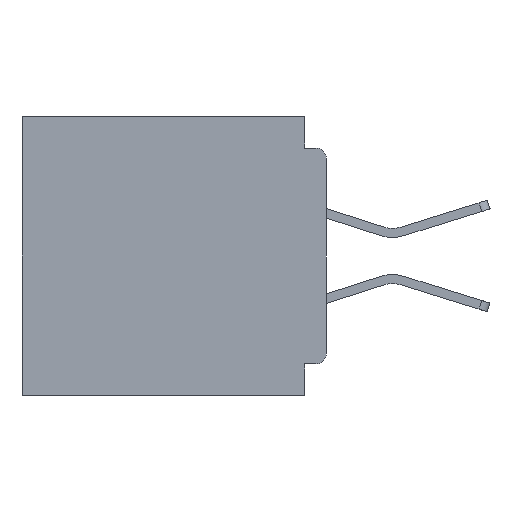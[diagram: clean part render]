
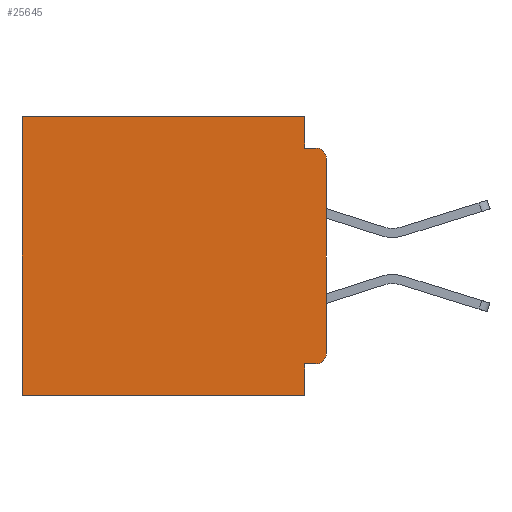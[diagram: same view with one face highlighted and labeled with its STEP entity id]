
A CAD part, left-side view. The second image highlights one B-rep face of the part: STEP entity #25645.
In plain terms, the highlighted planar face has unit normal (-1, 0, 0).
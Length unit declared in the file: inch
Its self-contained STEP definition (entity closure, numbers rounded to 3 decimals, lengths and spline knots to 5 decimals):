
#395 = FACE_OUTER_BOUND ( 'NONE', #23932, .T. ) ;
#599 = LINE ( 'NONE', #35341, #52289 ) ;
#626 = AXIS2_PLACEMENT_3D ( 'NONE', #2912, #31562, #7091 ) ;
#1434 = EDGE_CURVE ( 'NONE', #46200, #26288, #18118, .T. ) ;
#2071 = EDGE_CURVE ( 'NONE', #22953, #18484, #30755, .T. ) ;
#2912 = CARTESIAN_POINT ( 'NONE',  ( 0.3, 0.015, -0.34 ) ) ;
#4743 = ORIENTED_EDGE ( 'NONE', *, *, #30629, .F. ) ;
#5328 = VECTOR ( 'NONE', #30180, 39.37008 ) ;
#5553 = ORIENTED_EDGE ( 'NONE', *, *, #47998, .F. ) ;
#5701 = CARTESIAN_POINT ( 'NONE',  ( 0.3, 0.031, -0.4 ) ) ;
#6143 = CARTESIAN_POINT ( 'NONE',  ( 0.3, 0.015, -0.06 ) ) ;
#6847 = VERTEX_POINT ( 'NONE', #40837 ) ;
#6984 = CARTESIAN_POINT ( 'NONE',  ( 0.3, 0., -0.4 ) ) ;
#7091 = DIRECTION ( 'NONE',  ( 0., 0., -1. ) ) ;
#7437 = CARTESIAN_POINT ( 'NONE',  ( 0.3, 0., -0.355 ) ) ;
#8600 = DIRECTION ( 'NONE',  ( 0., 1., 0. ) ) ;
#8680 = VERTEX_POINT ( 'NONE', #18817 ) ;
#9049 = VERTEX_POINT ( 'NONE', #9084 ) ;
#9084 = CARTESIAN_POINT ( 'NONE',  ( 0.3, 0., -0.34 ) ) ;
#9316 = ORIENTED_EDGE ( 'NONE', *, *, #34991, .F. ) ;
#10979 = CARTESIAN_POINT ( 'NONE',  ( 0.3, 0.031, 0. ) ) ;
#11199 = LINE ( 'NONE', #37113, #43666 ) ;
#11327 = DIRECTION ( 'NONE',  ( 1., 0., 0. ) ) ;
#14167 = ORIENTED_EDGE ( 'NONE', *, *, #1434, .T. ) ;
#15067 = DIRECTION ( 'NONE',  ( 0., 0., -1. ) ) ;
#16096 = EDGE_CURVE ( 'NONE', #16670, #6847, #599, .T. ) ;
#16670 = VERTEX_POINT ( 'NONE', #30501 ) ;
#16871 = ORIENTED_EDGE ( 'NONE', *, *, #35372, .T. ) ;
#18118 = CIRCLE ( 'NONE', #34537, 0.015 ) ;
#18194 = LINE ( 'NONE', #7437, #39817 ) ;
#18484 = VERTEX_POINT ( 'NONE', #30684 ) ;
#18817 = CARTESIAN_POINT ( 'NONE',  ( 0.3, 0.031, -0.4 ) ) ;
#19223 = DIRECTION ( 'NONE',  ( 0., 0., -1. ) ) ;
#19970 = VECTOR ( 'NONE', #29148, 39.37008 ) ;
#20769 = EDGE_CURVE ( 'NONE', #34460, #38679, #18194, .T. ) ;
#20988 = CARTESIAN_POINT ( 'NONE',  ( 0.3, 0., -0.06 ) ) ;
#22665 = DIRECTION ( 'NONE',  ( 0., 1., 0. ) ) ;
#22953 = VERTEX_POINT ( 'NONE', #10979 ) ;
#23932 = EDGE_LOOP ( 'NONE', ( #4743, #14167, #5553, #24579, #46539, #24917, #9316, #52627, #30389, #16871 ) ) ;
#24579 = ORIENTED_EDGE ( 'NONE', *, *, #2071, .F. ) ;
#24917 = ORIENTED_EDGE ( 'NONE', *, *, #16096, .T. ) ;
#25645 = ADVANCED_FACE ( 'NONE', ( #395 ), #47808, .F. ) ;
#26288 = VERTEX_POINT ( 'NONE', #43817 ) ;
#29148 = DIRECTION ( 'NONE',  ( 0., 0., -1. ) ) ;
#30180 = DIRECTION ( 'NONE',  ( 0., 0., -1. ) ) ;
#30389 = ORIENTED_EDGE ( 'NONE', *, *, #20769, .F. ) ;
#30501 = CARTESIAN_POINT ( 'NONE',  ( 0.3, 0.437, 0. ) ) ;
#30554 = LINE ( 'NONE', #42719, #50867 ) ;
#30629 = EDGE_CURVE ( 'NONE', #46200, #9049, #50084, .T. ) ;
#30684 = CARTESIAN_POINT ( 'NONE',  ( 0.3, 0.031, -0.045 ) ) ;
#30755 = LINE ( 'NONE', #44254, #19970 ) ;
#31562 = DIRECTION ( 'NONE',  ( -1., 0., 0. ) ) ;
#33025 = LINE ( 'NONE', #47759, #52037 ) ;
#34109 = DIRECTION ( 'NONE',  ( 0., 0., -1. ) ) ;
#34460 = VERTEX_POINT ( 'NONE', #45673 ) ;
#34537 = AXIS2_PLACEMENT_3D ( 'NONE', #6143, #46191, #34109 ) ;
#34991 = EDGE_CURVE ( 'NONE', #8680, #6847, #11199, .T. ) ;
#35341 = CARTESIAN_POINT ( 'NONE',  ( 0.3, 0.437, -0.4 ) ) ;
#35357 = CIRCLE ( 'NONE', #626, 0.015 ) ;
#35372 = EDGE_CURVE ( 'NONE', #34460, #9049, #35357, .T. ) ;
#35495 = DIRECTION ( 'NONE',  ( 0., -1., 0. ) ) ;
#35719 = CARTESIAN_POINT ( 'NONE',  ( 0.3, 0., -0.4 ) ) ;
#36554 = CARTESIAN_POINT ( 'NONE',  ( 0.3, 0.031, -0.355 ) ) ;
#37113 = CARTESIAN_POINT ( 'NONE',  ( 0.3, 0., -0.4 ) ) ;
#38679 = VERTEX_POINT ( 'NONE', #36554 ) ;
#39811 = DIRECTION ( 'NONE',  ( 0., 0., -1. ) ) ;
#39817 = VECTOR ( 'NONE', #51951, 39.37008 ) ;
#40761 = AXIS2_PLACEMENT_3D ( 'NONE', #35719, #11327, #39811 ) ;
#40837 = CARTESIAN_POINT ( 'NONE',  ( 0.3, 0.437, -0.4 ) ) ;
#42719 = CARTESIAN_POINT ( 'NONE',  ( 0.3, 0., 0. ) ) ;
#43666 = VECTOR ( 'NONE', #8600, 39.37008 ) ;
#43817 = CARTESIAN_POINT ( 'NONE',  ( 0.3, 0.015, -0.045 ) ) ;
#44254 = CARTESIAN_POINT ( 'NONE',  ( 0.3, 0.031, 0. ) ) ;
#45673 = CARTESIAN_POINT ( 'NONE',  ( 0.3, 0.015, -0.355 ) ) ;
#46191 = DIRECTION ( 'NONE',  ( -1., 0., 0. ) ) ;
#46200 = VERTEX_POINT ( 'NONE', #20988 ) ;
#46539 = ORIENTED_EDGE ( 'NONE', *, *, #47170, .T. ) ;
#47170 = EDGE_CURVE ( 'NONE', #22953, #16670, #30554, .T. ) ;
#47759 = CARTESIAN_POINT ( 'NONE',  ( 0.3, 0., -0.045 ) ) ;
#47808 = PLANE ( 'NONE',  #40761 ) ;
#47998 = EDGE_CURVE ( 'NONE', #18484, #26288, #33025, .T. ) ;
#48720 = LINE ( 'NONE', #5701, #5328 ) ;
#48835 = VECTOR ( 'NONE', #19223, 39.37008 ) ;
#49630 = EDGE_CURVE ( 'NONE', #38679, #8680, #48720, .T. ) ;
#50084 = LINE ( 'NONE', #6984, #48835 ) ;
#50867 = VECTOR ( 'NONE', #22665, 39.37008 ) ;
#51951 = DIRECTION ( 'NONE',  ( 0., 1., 0. ) ) ;
#52037 = VECTOR ( 'NONE', #35495, 39.37008 ) ;
#52289 = VECTOR ( 'NONE', #15067, 39.37008 ) ;
#52627 = ORIENTED_EDGE ( 'NONE', *, *, #49630, .F. ) ;
